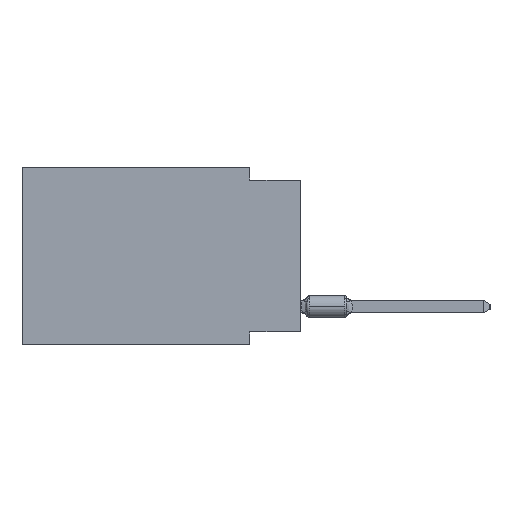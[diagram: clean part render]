
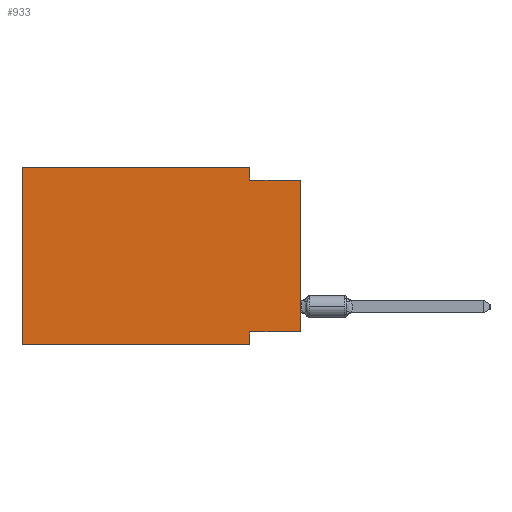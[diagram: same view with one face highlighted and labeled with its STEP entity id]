
A CAD part, left-side view. The second image highlights one B-rep face of the part: STEP entity #933.
In plain terms, the highlighted planar face has unit normal (-1, 0, 0).
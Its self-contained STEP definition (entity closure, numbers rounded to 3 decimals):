
#864 = CARTESIAN_POINT ( 'NONE',  ( 0., 0., -0.635 ) ) ;
#933 = ADVANCED_FACE ( 'NONE', ( #19670 ), #58467, .F. ) ;
#1681 = CARTESIAN_POINT ( 'NONE',  ( 0., 2.54, 0. ) ) ;
#1961 = DIRECTION ( 'NONE',  ( 1., 0., 0. ) ) ;
#3632 = CARTESIAN_POINT ( 'NONE',  ( 0., 13.97, -8.89 ) ) ;
#5681 = VECTOR ( 'NONE', #41512, 1000. ) ;
#5769 = VECTOR ( 'NONE', #40811, 1000. ) ;
#6154 = DIRECTION ( 'NONE',  ( 0., -1., 0. ) ) ;
#7947 = ORIENTED_EDGE ( 'NONE', *, *, #46886, .F. ) ;
#8040 = CARTESIAN_POINT ( 'NONE',  ( 0., 2.54, -8.89 ) ) ;
#11134 = EDGE_CURVE ( 'NONE', #12979, #49220, #49237, .T. ) ;
#12037 = ORIENTED_EDGE ( 'NONE', *, *, #25082, .F. ) ;
#12157 = CARTESIAN_POINT ( 'NONE',  ( 0., 0., -8.255 ) ) ;
#12752 = VECTOR ( 'NONE', #31319, 1000. ) ;
#12979 = VERTEX_POINT ( 'NONE', #21846 ) ;
#14006 = ORIENTED_EDGE ( 'NONE', *, *, #29960, .F. ) ;
#14228 = ORIENTED_EDGE ( 'NONE', *, *, #45890, .T. ) ;
#15405 = VERTEX_POINT ( 'NONE', #41342 ) ;
#16911 = LINE ( 'NONE', #35851, #5769 ) ;
#19253 = VECTOR ( 'NONE', #24741, 1000. ) ;
#19670 = FACE_OUTER_BOUND ( 'NONE', #23815, .T. ) ;
#20103 = CARTESIAN_POINT ( 'NONE',  ( 0., 13.97, 0. ) ) ;
#21326 = VECTOR ( 'NONE', #31102, 1000. ) ;
#21846 = CARTESIAN_POINT ( 'NONE',  ( 0., 0., -8.255 ) ) ;
#22329 = AXIS2_PLACEMENT_3D ( 'NONE', #29294, #1961, #30520 ) ;
#23815 = EDGE_LOOP ( 'NONE', ( #25313, #12037, #41005, #14006, #57747, #14228, #7947, #45640 ) ) ;
#24741 = DIRECTION ( 'NONE',  ( 0., 0., 1. ) ) ;
#25082 = EDGE_CURVE ( 'NONE', #35708, #49220, #39348, .T. ) ;
#25313 = ORIENTED_EDGE ( 'NONE', *, *, #11134, .T. ) ;
#25417 = VERTEX_POINT ( 'NONE', #57967 ) ;
#25978 = CARTESIAN_POINT ( 'NONE',  ( 0., 0., 0. ) ) ;
#26220 = CARTESIAN_POINT ( 'NONE',  ( 0., 13.97, 0. ) ) ;
#26397 = VERTEX_POINT ( 'NONE', #59357 ) ;
#26933 = CARTESIAN_POINT ( 'NONE',  ( 0., 0., -0.635 ) ) ;
#27217 = VECTOR ( 'NONE', #34701, 1000. ) ;
#27777 = VECTOR ( 'NONE', #6154, 1000. ) ;
#29294 = CARTESIAN_POINT ( 'NONE',  ( 0., 13.97, 0. ) ) ;
#29384 = EDGE_CURVE ( 'NONE', #12979, #15405, #40398, .T. ) ;
#29643 = DIRECTION ( 'NONE',  ( 0., 0., -1. ) ) ;
#29960 = EDGE_CURVE ( 'NONE', #42606, #26397, #48041, .T. ) ;
#30520 = DIRECTION ( 'NONE',  ( 0., 0., -1. ) ) ;
#31102 = DIRECTION ( 'NONE',  ( 0., 1., 0. ) ) ;
#31319 = DIRECTION ( 'NONE',  ( 0., 0., -1. ) ) ;
#34701 = DIRECTION ( 'NONE',  ( 0., -1., 0. ) ) ;
#35708 = VERTEX_POINT ( 'NONE', #55066 ) ;
#35851 = CARTESIAN_POINT ( 'NONE',  ( 0., 13.97, 0. ) ) ;
#39348 = LINE ( 'NONE', #864, #27777 ) ;
#40398 = LINE ( 'NONE', #12157, #21326 ) ;
#40811 = DIRECTION ( 'NONE',  ( 0., 0., 1. ) ) ;
#41005 = ORIENTED_EDGE ( 'NONE', *, *, #44458, .F. ) ;
#41342 = CARTESIAN_POINT ( 'NONE',  ( 0., 2.54, -8.255 ) ) ;
#41512 = DIRECTION ( 'NONE',  ( 0., -1., 0. ) ) ;
#42606 = VERTEX_POINT ( 'NONE', #26220 ) ;
#44458 = EDGE_CURVE ( 'NONE', #26397, #35708, #52926, .T. ) ;
#45640 = ORIENTED_EDGE ( 'NONE', *, *, #29384, .F. ) ;
#45890 = EDGE_CURVE ( 'NONE', #25417, #45933, #46168, .T. ) ;
#45933 = VERTEX_POINT ( 'NONE', #57317 ) ;
#46168 = LINE ( 'NONE', #3632, #5681 ) ;
#46886 = EDGE_CURVE ( 'NONE', #15405, #45933, #50564, .T. ) ;
#48041 = LINE ( 'NONE', #20103, #27217 ) ;
#49220 = VERTEX_POINT ( 'NONE', #26933 ) ;
#49237 = LINE ( 'NONE', #25978, #19253 ) ;
#50564 = LINE ( 'NONE', #8040, #12752 ) ;
#52926 = LINE ( 'NONE', #1681, #60425 ) ;
#55066 = CARTESIAN_POINT ( 'NONE',  ( 0., 2.54, -0.635 ) ) ;
#57317 = CARTESIAN_POINT ( 'NONE',  ( 0., 2.54, -8.89 ) ) ;
#57747 = ORIENTED_EDGE ( 'NONE', *, *, #59332, .F. ) ;
#57967 = CARTESIAN_POINT ( 'NONE',  ( 0., 13.97, -8.89 ) ) ;
#58467 = PLANE ( 'NONE',  #22329 ) ;
#59332 = EDGE_CURVE ( 'NONE', #25417, #42606, #16911, .T. ) ;
#59357 = CARTESIAN_POINT ( 'NONE',  ( 0., 2.54, 0. ) ) ;
#60425 = VECTOR ( 'NONE', #29643, 1000. ) ;
